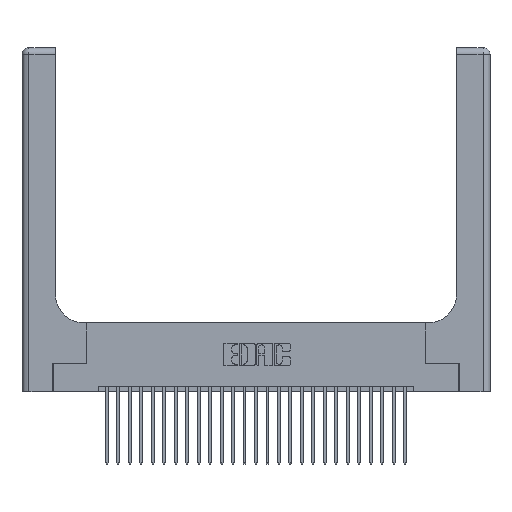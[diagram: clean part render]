
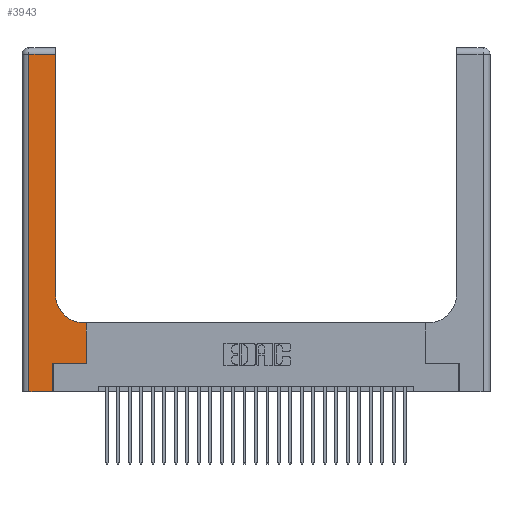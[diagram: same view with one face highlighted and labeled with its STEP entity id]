
A CAD part, top view. The second image highlights one B-rep face of the part: STEP entity #3943.
In plain terms, the highlighted planar face has unit normal (0, 0, 1).
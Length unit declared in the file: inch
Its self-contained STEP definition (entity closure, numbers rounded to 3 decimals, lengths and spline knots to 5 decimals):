
#498 = LINE ( 'NONE', #7965, #4599 ) ;
#538 = EDGE_CURVE ( 'NONE', #23154, #25103, #16123, .T. ) ;
#713 = CARTESIAN_POINT ( 'NONE',  ( 0.5415, 0.85, 0.37 ) ) ;
#1464 = VERTEX_POINT ( 'NONE', #18512 ) ;
#2665 = DIRECTION ( 'NONE',  ( -1., 0., 0. ) ) ;
#2807 = EDGE_CURVE ( 'NONE', #6937, #1464, #6060, .T. ) ;
#2931 = DIRECTION ( 'NONE',  ( 1., 0., 0. ) ) ;
#3017 = VECTOR ( 'NONE', #10764, 39.37008 ) ;
#3035 = LINE ( 'NONE', #13649, #4381 ) ;
#3868 = VERTEX_POINT ( 'NONE', #9560 ) ;
#3943 = ADVANCED_FACE ( 'NONE', ( #16653 ), #20453, .F. ) ;
#4381 = VECTOR ( 'NONE', #24749, 39.37008 ) ;
#4599 = VECTOR ( 'NONE', #5652, 39.37008 ) ;
#4886 = EDGE_CURVE ( 'NONE', #3868, #27186, #20071, .T. ) ;
#5107 = CARTESIAN_POINT ( 'NONE',  ( 0.06, 0., 0.37 ) ) ;
#5242 = CARTESIAN_POINT ( 'NONE',  ( 0., 3., 0.37 ) ) ;
#5652 = DIRECTION ( 'NONE',  ( 1., 0., 0. ) ) ;
#5800 = CARTESIAN_POINT ( 'NONE',  ( 0.5585, 0.25, 0.37 ) ) ;
#5809 = ORIENTED_EDGE ( 'NONE', *, *, #10960, .T. ) ;
#5914 = EDGE_CURVE ( 'NONE', #25103, #3868, #15824, .T. ) ;
#6060 = LINE ( 'NONE', #25557, #3017 ) ;
#6388 = EDGE_CURVE ( 'NONE', #27186, #6937, #21704, .T. ) ;
#6937 = VERTEX_POINT ( 'NONE', #25496 ) ;
#7264 = VECTOR ( 'NONE', #2665, 39.37008 ) ;
#7609 = VECTOR ( 'NONE', #18188, 39.37008 ) ;
#7691 = DIRECTION ( 'NONE',  ( 1., 0., 0. ) ) ;
#7870 = CARTESIAN_POINT ( 'NONE',  ( 0.269, 0., 0.37 ) ) ;
#7965 = CARTESIAN_POINT ( 'NONE',  ( 0., 0., 0.37 ) ) ;
#9560 = CARTESIAN_POINT ( 'NONE',  ( 0.5415, 0.6, 0.37 ) ) ;
#9656 = LINE ( 'NONE', #7870, #24440 ) ;
#10269 = VERTEX_POINT ( 'NONE', #5107 ) ;
#10296 = VECTOR ( 'NONE', #25790, 39.37008 ) ;
#10608 = ORIENTED_EDGE ( 'NONE', *, *, #2807, .T. ) ;
#10764 = DIRECTION ( 'NONE',  ( -1., 0., 0. ) ) ;
#10960 = EDGE_CURVE ( 'NONE', #10269, #12969, #498, .T. ) ;
#11961 = ORIENTED_EDGE ( 'NONE', *, *, #4886, .T. ) ;
#12572 = VECTOR ( 'NONE', #7691, 39.37008 ) ;
#12786 = CARTESIAN_POINT ( 'NONE',  ( 0.2915, 0.85, 0.37 ) ) ;
#12857 = EDGE_CURVE ( 'NONE', #12969, #13414, #9656, .T. ) ;
#12969 = VERTEX_POINT ( 'NONE', #15005 ) ;
#13414 = VERTEX_POINT ( 'NONE', #26910 ) ;
#13649 = CARTESIAN_POINT ( 'NONE',  ( 0.06, 3., 0.37 ) ) ;
#13853 = DIRECTION ( 'NONE',  ( 0., 0., -1. ) ) ;
#14465 = DIRECTION ( 'NONE',  ( 0., 1., 0. ) ) ;
#15005 = CARTESIAN_POINT ( 'NONE',  ( 0.269, 0., 0.37 ) ) ;
#15750 = CARTESIAN_POINT ( 'NONE',  ( 0.2915, 0.6, 0.37 ) ) ;
#15824 = LINE ( 'NONE', #15750, #7264 ) ;
#16018 = CARTESIAN_POINT ( 'NONE',  ( 0.5585, 0.25, 0.37 ) ) ;
#16020 = DIRECTION ( 'NONE',  ( 0., 0., -1. ) ) ;
#16123 = LINE ( 'NONE', #5800, #10296 ) ;
#16441 = ORIENTED_EDGE ( 'NONE', *, *, #24867, .T. ) ;
#16653 = FACE_OUTER_BOUND ( 'NONE', #26766, .T. ) ;
#17046 = EDGE_CURVE ( 'NONE', #13414, #23154, #21209, .T. ) ;
#17568 = ORIENTED_EDGE ( 'NONE', *, *, #5914, .T. ) ;
#18188 = DIRECTION ( 'NONE',  ( 0., 1., 0. ) ) ;
#18384 = DIRECTION ( 'NONE',  ( -1., 0., 0. ) ) ;
#18512 = CARTESIAN_POINT ( 'NONE',  ( 0.06, 2.94, 0.37 ) ) ;
#18853 = ORIENTED_EDGE ( 'NONE', *, *, #12857, .T. ) ;
#19088 = ORIENTED_EDGE ( 'NONE', *, *, #6388, .T. ) ;
#20071 = CIRCLE ( 'NONE', #24110, 0.25 ) ;
#20453 = PLANE ( 'NONE',  #25189 ) ;
#20850 = CARTESIAN_POINT ( 'NONE',  ( 0.269, 0.25, 0.37 ) ) ;
#21209 = LINE ( 'NONE', #20850, #12572 ) ;
#21704 = LINE ( 'NONE', #27687, #7609 ) ;
#23154 = VERTEX_POINT ( 'NONE', #16018 ) ;
#23412 = CARTESIAN_POINT ( 'NONE',  ( 0.5585, 0.6, 0.37 ) ) ;
#24110 = AXIS2_PLACEMENT_3D ( 'NONE', #713, #16020, #2931 ) ;
#24440 = VECTOR ( 'NONE', #14465, 39.37008 ) ;
#24749 = DIRECTION ( 'NONE',  ( 0., -1., 0. ) ) ;
#24867 = EDGE_CURVE ( 'NONE', #1464, #10269, #3035, .T. ) ;
#25103 = VERTEX_POINT ( 'NONE', #23412 ) ;
#25189 = AXIS2_PLACEMENT_3D ( 'NONE', #5242, #13853, #18384 ) ;
#25496 = CARTESIAN_POINT ( 'NONE',  ( 0.2915, 2.94, 0.37 ) ) ;
#25557 = CARTESIAN_POINT ( 'NONE',  ( 0., 2.94, 0.37 ) ) ;
#25629 = ORIENTED_EDGE ( 'NONE', *, *, #538, .T. ) ;
#25790 = DIRECTION ( 'NONE',  ( 0., 1., 0. ) ) ;
#26766 = EDGE_LOOP ( 'NONE', ( #19088, #10608, #16441, #5809, #18853, #28283, #25629, #17568, #11961 ) ) ;
#26910 = CARTESIAN_POINT ( 'NONE',  ( 0.269, 0.25, 0.37 ) ) ;
#27186 = VERTEX_POINT ( 'NONE', #12786 ) ;
#27687 = CARTESIAN_POINT ( 'NONE',  ( 0.2915, 3., 0.37 ) ) ;
#28283 = ORIENTED_EDGE ( 'NONE', *, *, #17046, .T. ) ;
